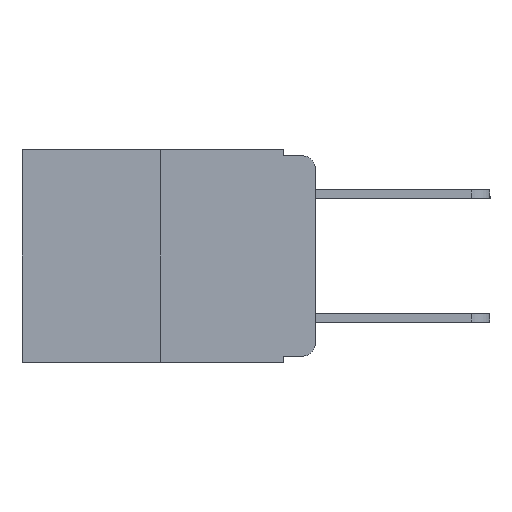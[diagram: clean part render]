
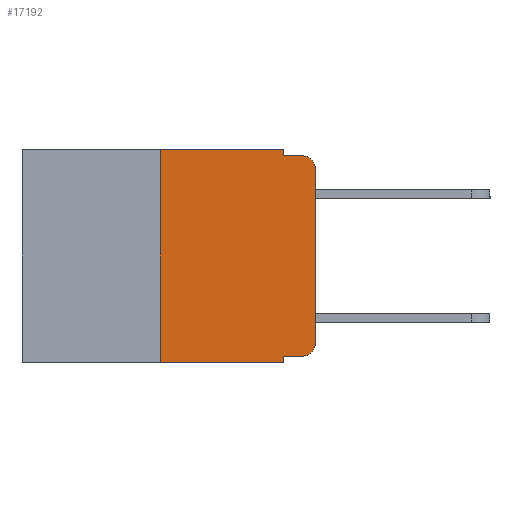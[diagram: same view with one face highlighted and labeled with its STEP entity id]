
A CAD part, left-side view. The second image highlights one B-rep face of the part: STEP entity #17192.
In plain terms, the highlighted planar face has unit normal (-1, 0, 0).
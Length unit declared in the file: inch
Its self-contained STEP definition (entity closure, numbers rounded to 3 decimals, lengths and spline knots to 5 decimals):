
#560 = LINE ( 'NONE', #19852, #16148 ) ;
#1195 = VECTOR ( 'NONE', #20049, 39.37008 ) ;
#1356 = VERTEX_POINT ( 'NONE', #9760 ) ;
#1867 = CARTESIAN_POINT ( 'NONE',  ( 0., 0.25, 0. ) ) ;
#2018 = VECTOR ( 'NONE', #23767, 39.37008 ) ;
#2038 = CARTESIAN_POINT ( 'NONE',  ( 0., 0.051, -0.01 ) ) ;
#2508 = ORIENTED_EDGE ( 'NONE', *, *, #7357, .F. ) ;
#2617 = EDGE_CURVE ( 'NONE', #14022, #1356, #24253, .T. ) ;
#2676 = LINE ( 'NONE', #12091, #2018 ) ;
#2730 = DIRECTION ( 'NONE',  ( 0., 0., 1. ) ) ;
#2943 = VERTEX_POINT ( 'NONE', #2038 ) ;
#3157 = EDGE_CURVE ( 'NONE', #9366, #2943, #17904, .T. ) ;
#3352 = CARTESIAN_POINT ( 'NONE',  ( 0., 0.473, 0. ) ) ;
#4637 = CARTESIAN_POINT ( 'NONE',  ( 0., 0.051, 0. ) ) ;
#5980 = EDGE_LOOP ( 'NONE', ( #17871, #13836, #2508, #15192, #21898, #23674, #25147, #14862, #9011, #11460 ) ) ;
#6104 = VECTOR ( 'NONE', #18699, 39.37008 ) ;
#6494 = VERTEX_POINT ( 'NONE', #10929 ) ;
#6654 = DIRECTION ( 'NONE',  ( 1., 0., 0. ) ) ;
#7357 = EDGE_CURVE ( 'NONE', #2943, #6494, #560, .T. ) ;
#7747 = AXIS2_PLACEMENT_3D ( 'NONE', #21260, #9512, #23170 ) ;
#8664 = VECTOR ( 'NONE', #13580, 39.37008 ) ;
#8723 = EDGE_CURVE ( 'NONE', #14022, #14754, #22467, .T. ) ;
#9001 = VERTEX_POINT ( 'NONE', #21418 ) ;
#9011 = ORIENTED_EDGE ( 'NONE', *, *, #2617, .T. ) ;
#9140 = VERTEX_POINT ( 'NONE', #10082 ) ;
#9366 = VERTEX_POINT ( 'NONE', #12808 ) ;
#9486 = LINE ( 'NONE', #12863, #19909 ) ;
#9512 = DIRECTION ( 'NONE',  ( -1., 0., 0. ) ) ;
#9755 = CARTESIAN_POINT ( 'NONE',  ( 0., 0.25, 0. ) ) ;
#9760 = CARTESIAN_POINT ( 'NONE',  ( 0., 0.02, -0.333 ) ) ;
#10082 = CARTESIAN_POINT ( 'NONE',  ( 0., 0.25, -0.343 ) ) ;
#10279 = FACE_OUTER_BOUND ( 'NONE', #5980, .T. ) ;
#10439 = VECTOR ( 'NONE', #24774, 39.37008 ) ;
#10929 = CARTESIAN_POINT ( 'NONE',  ( 0., 0.02, -0.01 ) ) ;
#11460 = ORIENTED_EDGE ( 'NONE', *, *, #23964, .T. ) ;
#11583 = VERTEX_POINT ( 'NONE', #21430 ) ;
#11990 = DIRECTION ( 'NONE',  ( -1., 0., 0. ) ) ;
#12091 = CARTESIAN_POINT ( 'NONE',  ( 0., 0.473, 0. ) ) ;
#12632 = VECTOR ( 'NONE', #22116, 39.37008 ) ;
#12808 = CARTESIAN_POINT ( 'NONE',  ( 0., 0.051, 0. ) ) ;
#12863 = CARTESIAN_POINT ( 'NONE',  ( 0., 0., 0. ) ) ;
#13050 = AXIS2_PLACEMENT_3D ( 'NONE', #3352, #6654, #16281 ) ;
#13258 = CARTESIAN_POINT ( 'NONE',  ( 0., 0.051, -0.333 ) ) ;
#13318 = LINE ( 'NONE', #1867, #1195 ) ;
#13320 = EDGE_CURVE ( 'NONE', #9140, #14754, #16296, .T. ) ;
#13467 = CARTESIAN_POINT ( 'NONE',  ( 0., 0.051, -0.343 ) ) ;
#13580 = DIRECTION ( 'NONE',  ( 0., -1., 0. ) ) ;
#13626 = EDGE_CURVE ( 'NONE', #14126, #9366, #2676, .T. ) ;
#13836 = ORIENTED_EDGE ( 'NONE', *, *, #17155, .T. ) ;
#14022 = VERTEX_POINT ( 'NONE', #13258 ) ;
#14126 = VERTEX_POINT ( 'NONE', #9755 ) ;
#14754 = VERTEX_POINT ( 'NONE', #13467 ) ;
#14862 = ORIENTED_EDGE ( 'NONE', *, *, #8723, .F. ) ;
#15192 = ORIENTED_EDGE ( 'NONE', *, *, #3157, .F. ) ;
#15538 = CARTESIAN_POINT ( 'NONE',  ( 0., 0.051, 0. ) ) ;
#16148 = VECTOR ( 'NONE', #21806, 39.37008 ) ;
#16208 = CARTESIAN_POINT ( 'NONE',  ( 0., 0.051, -0.333 ) ) ;
#16281 = DIRECTION ( 'NONE',  ( 0., 0., -1. ) ) ;
#16296 = LINE ( 'NONE', #21019, #10439 ) ;
#17155 = EDGE_CURVE ( 'NONE', #11583, #6494, #24602, .T. ) ;
#17162 = CIRCLE ( 'NONE', #25354, 0.02 ) ;
#17192 = ADVANCED_FACE ( 'NONE', ( #10279 ), #23249, .F. ) ;
#17871 = ORIENTED_EDGE ( 'NONE', *, *, #23634, .T. ) ;
#17904 = LINE ( 'NONE', #15538, #12632 ) ;
#18699 = DIRECTION ( 'NONE',  ( 0., 0., -1. ) ) ;
#19852 = CARTESIAN_POINT ( 'NONE',  ( 0., 0.051, -0.01 ) ) ;
#19909 = VECTOR ( 'NONE', #2730, 39.37008 ) ;
#20049 = DIRECTION ( 'NONE',  ( 0., 0., 1. ) ) ;
#20575 = EDGE_CURVE ( 'NONE', #9140, #14126, #13318, .T. ) ;
#21019 = CARTESIAN_POINT ( 'NONE',  ( 0., 0.473, -0.343 ) ) ;
#21260 = CARTESIAN_POINT ( 'NONE',  ( 0., 0.02, -0.03 ) ) ;
#21418 = CARTESIAN_POINT ( 'NONE',  ( 0., 0., -0.313 ) ) ;
#21430 = CARTESIAN_POINT ( 'NONE',  ( 0., 0., -0.03 ) ) ;
#21806 = DIRECTION ( 'NONE',  ( 0., -1., 0. ) ) ;
#21898 = ORIENTED_EDGE ( 'NONE', *, *, #13626, .F. ) ;
#22116 = DIRECTION ( 'NONE',  ( 0., 0., -1. ) ) ;
#22467 = LINE ( 'NONE', #4637, #6104 ) ;
#23170 = DIRECTION ( 'NONE',  ( 0., 0., -1. ) ) ;
#23249 = PLANE ( 'NONE',  #13050 ) ;
#23634 = EDGE_CURVE ( 'NONE', #9001, #11583, #9486, .T. ) ;
#23674 = ORIENTED_EDGE ( 'NONE', *, *, #20575, .F. ) ;
#23688 = CARTESIAN_POINT ( 'NONE',  ( 0., 0.02, -0.313 ) ) ;
#23767 = DIRECTION ( 'NONE',  ( 0., -1., 0. ) ) ;
#23964 = EDGE_CURVE ( 'NONE', #1356, #9001, #17162, .T. ) ;
#24253 = LINE ( 'NONE', #16208, #8664 ) ;
#24602 = CIRCLE ( 'NONE', #7747, 0.02 ) ;
#24774 = DIRECTION ( 'NONE',  ( 0., -1., 0. ) ) ;
#25147 = ORIENTED_EDGE ( 'NONE', *, *, #13320, .T. ) ;
#25354 = AXIS2_PLACEMENT_3D ( 'NONE', #23688, #11990, #25578 ) ;
#25578 = DIRECTION ( 'NONE',  ( 0., 0., -1. ) ) ;
